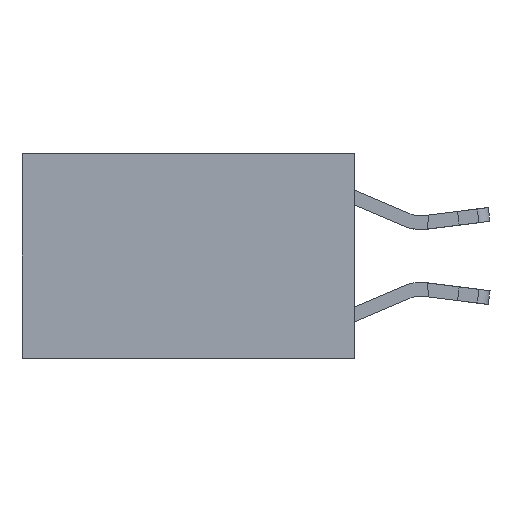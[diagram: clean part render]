
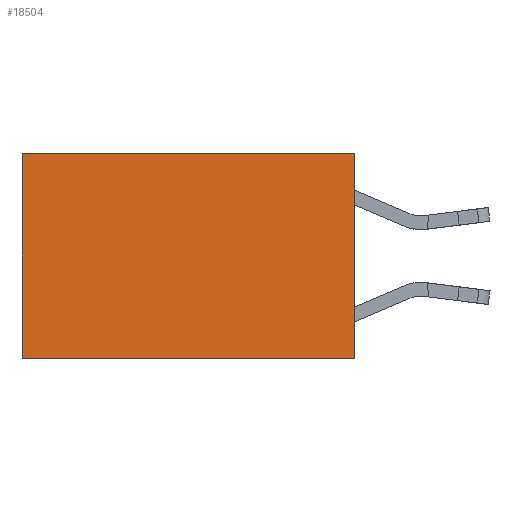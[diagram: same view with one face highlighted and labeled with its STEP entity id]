
A CAD part, left-side view. The second image highlights one B-rep face of the part: STEP entity #18504.
In plain terms, the highlighted planar face has unit normal (-1, 0, 0).
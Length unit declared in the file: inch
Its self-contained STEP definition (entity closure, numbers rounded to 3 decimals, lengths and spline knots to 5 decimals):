
#370 = EDGE_LOOP ( 'NONE', ( #17712, #2304, #13020, #17253 ) ) ;
#663 = FACE_OUTER_BOUND ( 'NONE', #370, .T. ) ;
#1080 = VERTEX_POINT ( 'NONE', #9262 ) ;
#1195 = DIRECTION ( 'NONE',  ( 0., 0., -1. ) ) ;
#1675 = LINE ( 'NONE', #16507, #5201 ) ;
#2304 = ORIENTED_EDGE ( 'NONE', *, *, #13328, .F. ) ;
#3784 = VERTEX_POINT ( 'NONE', #20849 ) ;
#3798 = VERTEX_POINT ( 'NONE', #9277 ) ;
#4562 = EDGE_CURVE ( 'NONE', #3784, #1080, #1675, .T. ) ;
#5201 = VECTOR ( 'NONE', #11425, 39.37008 ) ;
#8016 = PLANE ( 'NONE',  #19781 ) ;
#8029 = CARTESIAN_POINT ( 'NONE',  ( 0.2625, 0., -0.37 ) ) ;
#9262 = CARTESIAN_POINT ( 'NONE',  ( 0.2625, 0.6, -0.37 ) ) ;
#9277 = CARTESIAN_POINT ( 'NONE',  ( 0.2625, 0., 0. ) ) ;
#9412 = VECTOR ( 'NONE', #19698, 39.37008 ) ;
#10333 = VERTEX_POINT ( 'NONE', #8029 ) ;
#11257 = EDGE_CURVE ( 'NONE', #3798, #10333, #15459, .T. ) ;
#11378 = DIRECTION ( 'NONE',  ( 1., 0., 0. ) ) ;
#11425 = DIRECTION ( 'NONE',  ( 0., 0., -1. ) ) ;
#11578 = CARTESIAN_POINT ( 'NONE',  ( 0.2625, 0., 0. ) ) ;
#13020 = ORIENTED_EDGE ( 'NONE', *, *, #11257, .F. ) ;
#13328 = EDGE_CURVE ( 'NONE', #10333, #1080, #15631, .T. ) ;
#13901 = LINE ( 'NONE', #18038, #9412 ) ;
#14055 = VECTOR ( 'NONE', #19942, 39.37008 ) ;
#14999 = CARTESIAN_POINT ( 'NONE',  ( 0.2625, 0., -0.37 ) ) ;
#15459 = LINE ( 'NONE', #11578, #19308 ) ;
#15631 = LINE ( 'NONE', #14999, #14055 ) ;
#16507 = CARTESIAN_POINT ( 'NONE',  ( 0.2625, 0.6, 0. ) ) ;
#17253 = ORIENTED_EDGE ( 'NONE', *, *, #19856, .T. ) ;
#17712 = ORIENTED_EDGE ( 'NONE', *, *, #4562, .T. ) ;
#18038 = CARTESIAN_POINT ( 'NONE',  ( 0.2625, 0., 0. ) ) ;
#18504 = ADVANCED_FACE ( 'NONE', ( #663 ), #8016, .F. ) ;
#19308 = VECTOR ( 'NONE', #21527, 39.37008 ) ;
#19667 = CARTESIAN_POINT ( 'NONE',  ( 0.2625, 0., 0. ) ) ;
#19698 = DIRECTION ( 'NONE',  ( 0., 1., 0. ) ) ;
#19781 = AXIS2_PLACEMENT_3D ( 'NONE', #19667, #11378, #1195 ) ;
#19856 = EDGE_CURVE ( 'NONE', #3798, #3784, #13901, .T. ) ;
#19942 = DIRECTION ( 'NONE',  ( 0., 1., 0. ) ) ;
#20849 = CARTESIAN_POINT ( 'NONE',  ( 0.2625, 0.6, 0. ) ) ;
#21527 = DIRECTION ( 'NONE',  ( 0., 0., -1. ) ) ;
